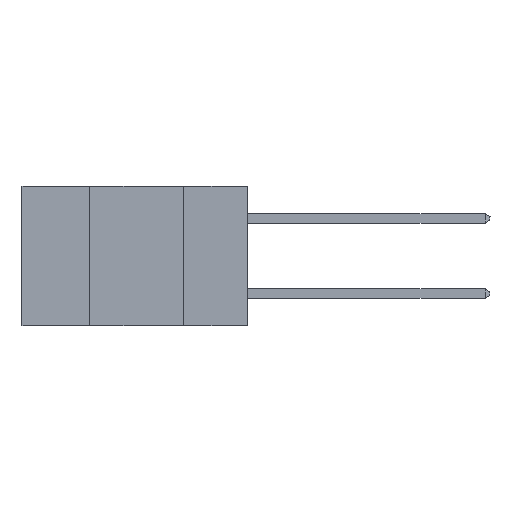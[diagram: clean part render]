
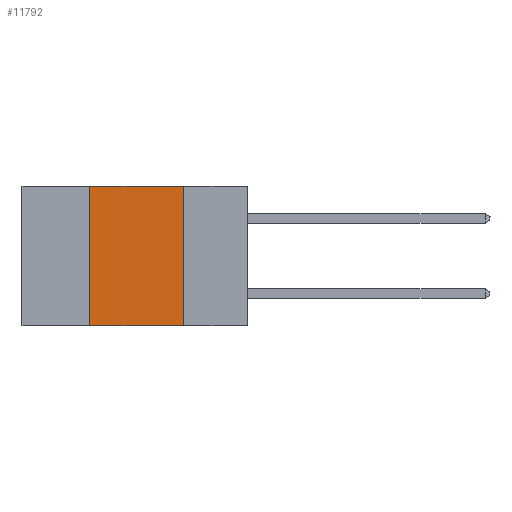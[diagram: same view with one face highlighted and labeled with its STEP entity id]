
A CAD part, left-side view. The second image highlights one B-rep face of the part: STEP entity #11792.
In plain terms, the highlighted planar face has unit normal (-1, 0, 0).
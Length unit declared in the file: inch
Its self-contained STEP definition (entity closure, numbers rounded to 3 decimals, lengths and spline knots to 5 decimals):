
#179 = VECTOR ( 'NONE', #26420, 39.37008 ) ;
#1144 = FACE_OUTER_BOUND ( 'NONE', #21263, .T. ) ;
#3325 = VECTOR ( 'NONE', #6444, 39.37008 ) ;
#4444 = CARTESIAN_POINT ( 'NONE',  ( 0., 0.17, 0. ) ) ;
#5108 = DIRECTION ( 'NONE',  ( 0., 0., -1. ) ) ;
#6444 = DIRECTION ( 'NONE',  ( 0., -1., 0. ) ) ;
#6450 = LINE ( 'NONE', #4444, #11119 ) ;
#7246 = VECTOR ( 'NONE', #25773, 39.37008 ) ;
#8489 = DIRECTION ( 'NONE',  ( 0., 0., -1. ) ) ;
#11119 = VECTOR ( 'NONE', #8489, 39.37008 ) ;
#11143 = CARTESIAN_POINT ( 'NONE',  ( 0., 0.17, 0. ) ) ;
#11521 = AXIS2_PLACEMENT_3D ( 'NONE', #22417, #11789, #5108 ) ;
#11789 = DIRECTION ( 'NONE',  ( 1., 0., 0. ) ) ;
#11792 = ADVANCED_FACE ( 'NONE', ( #1144 ), #15947, .F. ) ;
#11829 = EDGE_CURVE ( 'NONE', #21769, #26750, #12161, .T. ) ;
#12161 = LINE ( 'NONE', #26314, #179 ) ;
#12813 = ORIENTED_EDGE ( 'NONE', *, *, #24526, .F. ) ;
#12931 = CARTESIAN_POINT ( 'NONE',  ( 0., 0.6, -0.37 ) ) ;
#13202 = CARTESIAN_POINT ( 'NONE',  ( 0., 0.17, -0.37 ) ) ;
#13615 = LINE ( 'NONE', #14888, #3325 ) ;
#13765 = CARTESIAN_POINT ( 'NONE',  ( 0., 0.42, 0. ) ) ;
#14282 = VERTEX_POINT ( 'NONE', #11143 ) ;
#14888 = CARTESIAN_POINT ( 'NONE',  ( 0., 0.6, 0. ) ) ;
#14942 = EDGE_CURVE ( 'NONE', #21769, #24785, #20607, .T. ) ;
#15947 = PLANE ( 'NONE',  #11521 ) ;
#18355 = ORIENTED_EDGE ( 'NONE', *, *, #14942, .T. ) ;
#19409 = ORIENTED_EDGE ( 'NONE', *, *, #26533, .F. ) ;
#20607 = LINE ( 'NONE', #12931, #7246 ) ;
#21263 = EDGE_LOOP ( 'NONE', ( #19409, #12813, #23968, #18355 ) ) ;
#21769 = VERTEX_POINT ( 'NONE', #23483 ) ;
#22417 = CARTESIAN_POINT ( 'NONE',  ( 0., 0.6, 0. ) ) ;
#23483 = CARTESIAN_POINT ( 'NONE',  ( 0., 0.42, -0.37 ) ) ;
#23968 = ORIENTED_EDGE ( 'NONE', *, *, #11829, .F. ) ;
#24526 = EDGE_CURVE ( 'NONE', #26750, #14282, #13615, .T. ) ;
#24785 = VERTEX_POINT ( 'NONE', #13202 ) ;
#25773 = DIRECTION ( 'NONE',  ( 0., -1., 0. ) ) ;
#26314 = CARTESIAN_POINT ( 'NONE',  ( 0., 0.42, 0. ) ) ;
#26420 = DIRECTION ( 'NONE',  ( 0., 0., 1. ) ) ;
#26533 = EDGE_CURVE ( 'NONE', #14282, #24785, #6450, .T. ) ;
#26750 = VERTEX_POINT ( 'NONE', #13765 ) ;
